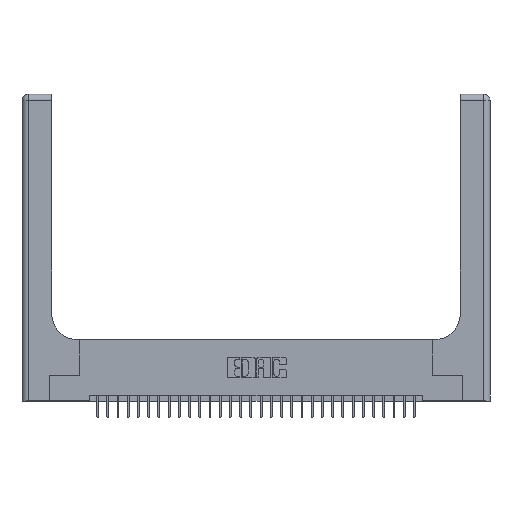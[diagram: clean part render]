
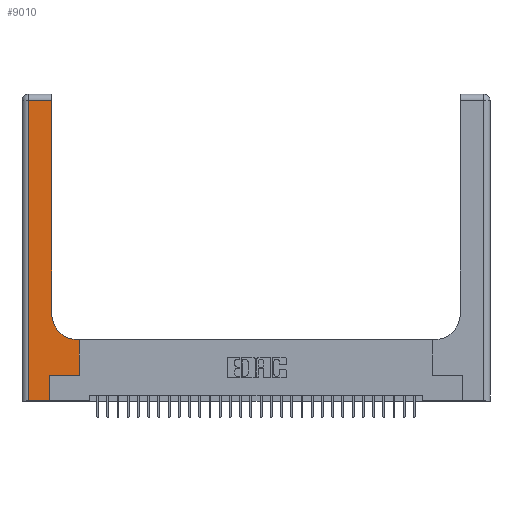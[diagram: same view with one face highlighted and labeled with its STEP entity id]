
A CAD part, top view. The second image highlights one B-rep face of the part: STEP entity #9010.
In plain terms, the highlighted planar face has unit normal (0, 0, 1).
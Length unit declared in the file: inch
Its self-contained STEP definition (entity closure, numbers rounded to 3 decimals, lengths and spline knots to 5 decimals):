
#358 = EDGE_CURVE ( 'NONE', #5891, #13282, #8172, .T. ) ;
#668 = DIRECTION ( 'NONE',  ( 0., 0., -1. ) ) ;
#2065 = DIRECTION ( 'NONE',  ( 1., 0., 0. ) ) ;
#2071 = ORIENTED_EDGE ( 'NONE', *, *, #5313, .T. ) ;
#2123 = AXIS2_PLACEMENT_3D ( 'NONE', #15393, #668, #19780 ) ;
#2156 = CARTESIAN_POINT ( 'NONE',  ( 0.269, 0., 0.37 ) ) ;
#2486 = EDGE_CURVE ( 'NONE', #23653, #8554, #8502, .T. ) ;
#2620 = LINE ( 'NONE', #26091, #23700 ) ;
#3602 = ORIENTED_EDGE ( 'NONE', *, *, #13614, .T. ) ;
#3738 = VECTOR ( 'NONE', #6688, 39.37008 ) ;
#3901 = EDGE_LOOP ( 'NONE', ( #3602, #21259, #10520, #13388, #2071, #23521, #14145, #7684, #25994 ) ) ;
#5313 = EDGE_CURVE ( 'NONE', #19761, #6849, #10259, .T. ) ;
#5891 = VERTEX_POINT ( 'NONE', #29740 ) ;
#6205 = VECTOR ( 'NONE', #19482, 39.37008 ) ;
#6592 = EDGE_CURVE ( 'NONE', #21903, #19761, #31597, .T. ) ;
#6688 = DIRECTION ( 'NONE',  ( 0., 1., 0. ) ) ;
#6849 = VERTEX_POINT ( 'NONE', #29167 ) ;
#7684 = ORIENTED_EDGE ( 'NONE', *, *, #17314, .T. ) ;
#8123 = VECTOR ( 'NONE', #10813, 39.37008 ) ;
#8172 = LINE ( 'NONE', #24734, #28862 ) ;
#8502 = LINE ( 'NONE', #12874, #8123 ) ;
#8554 = VERTEX_POINT ( 'NONE', #19736 ) ;
#9010 = ADVANCED_FACE ( 'NONE', ( #29563 ), #10465, .F. ) ;
#9840 = CARTESIAN_POINT ( 'NONE',  ( 0.269, 0., 0.37 ) ) ;
#10122 = EDGE_CURVE ( 'NONE', #13282, #21903, #19143, .T. ) ;
#10259 = LINE ( 'NONE', #2156, #3738 ) ;
#10278 = CARTESIAN_POINT ( 'NONE',  ( 0.2915, 3., 0.37 ) ) ;
#10465 = PLANE ( 'NONE',  #2123 ) ;
#10520 = ORIENTED_EDGE ( 'NONE', *, *, #10122, .T. ) ;
#10813 = DIRECTION ( 'NONE',  ( 0., 1., 0. ) ) ;
#11694 = DIRECTION ( 'NONE',  ( 1., 0., 0. ) ) ;
#12305 = CARTESIAN_POINT ( 'NONE',  ( 0.06, 3., 0.37 ) ) ;
#12601 = LINE ( 'NONE', #10278, #27867 ) ;
#12874 = CARTESIAN_POINT ( 'NONE',  ( 0.5585, 0.25, 0.37 ) ) ;
#13282 = VERTEX_POINT ( 'NONE', #31116 ) ;
#13388 = ORIENTED_EDGE ( 'NONE', *, *, #6592, .T. ) ;
#13614 = EDGE_CURVE ( 'NONE', #23960, #5891, #12601, .T. ) ;
#13869 = EDGE_CURVE ( 'NONE', #16204, #23960, #15624, .T. ) ;
#14003 = VECTOR ( 'NONE', #16223, 39.37008 ) ;
#14145 = ORIENTED_EDGE ( 'NONE', *, *, #2486, .T. ) ;
#14437 = CARTESIAN_POINT ( 'NONE',  ( 0.5415, 0.85, 0.37 ) ) ;
#15393 = CARTESIAN_POINT ( 'NONE',  ( 0., 3., 0.37 ) ) ;
#15423 = LINE ( 'NONE', #22068, #6205 ) ;
#15624 = CIRCLE ( 'NONE', #28892, 0.25 ) ;
#16204 = VERTEX_POINT ( 'NONE', #20598 ) ;
#16223 = DIRECTION ( 'NONE',  ( 1., 0., 0. ) ) ;
#16461 = VECTOR ( 'NONE', #17205, 39.37008 ) ;
#16772 = DIRECTION ( 'NONE',  ( 0., 0., -1. ) ) ;
#17205 = DIRECTION ( 'NONE',  ( 0., -1., 0. ) ) ;
#17314 = EDGE_CURVE ( 'NONE', #8554, #16204, #15423, .T. ) ;
#18265 = CARTESIAN_POINT ( 'NONE',  ( 0.2915, 0.85, 0.37 ) ) ;
#18275 = DIRECTION ( 'NONE',  ( 0., 1., 0. ) ) ;
#19143 = LINE ( 'NONE', #12305, #16461 ) ;
#19157 = EDGE_CURVE ( 'NONE', #6849, #23653, #2620, .T. ) ;
#19482 = DIRECTION ( 'NONE',  ( -1., 0., 0. ) ) ;
#19736 = CARTESIAN_POINT ( 'NONE',  ( 0.5585, 0.6, 0.37 ) ) ;
#19761 = VERTEX_POINT ( 'NONE', #9840 ) ;
#19780 = DIRECTION ( 'NONE',  ( -1., 0., 0. ) ) ;
#20598 = CARTESIAN_POINT ( 'NONE',  ( 0.5415, 0.6, 0.37 ) ) ;
#20725 = CARTESIAN_POINT ( 'NONE',  ( 0., 0., 0.37 ) ) ;
#21259 = ORIENTED_EDGE ( 'NONE', *, *, #358, .T. ) ;
#21903 = VERTEX_POINT ( 'NONE', #26254 ) ;
#22068 = CARTESIAN_POINT ( 'NONE',  ( 0.2915, 0.6, 0.37 ) ) ;
#23521 = ORIENTED_EDGE ( 'NONE', *, *, #19157, .T. ) ;
#23653 = VERTEX_POINT ( 'NONE', #29015 ) ;
#23700 = VECTOR ( 'NONE', #11694, 39.37008 ) ;
#23960 = VERTEX_POINT ( 'NONE', #18265 ) ;
#24734 = CARTESIAN_POINT ( 'NONE',  ( 0., 2.94, 0.37 ) ) ;
#25994 = ORIENTED_EDGE ( 'NONE', *, *, #13869, .T. ) ;
#26091 = CARTESIAN_POINT ( 'NONE',  ( 0.269, 0.25, 0.37 ) ) ;
#26254 = CARTESIAN_POINT ( 'NONE',  ( 0.06, 0., 0.37 ) ) ;
#27867 = VECTOR ( 'NONE', #18275, 39.37008 ) ;
#28862 = VECTOR ( 'NONE', #29356, 39.37008 ) ;
#28892 = AXIS2_PLACEMENT_3D ( 'NONE', #14437, #16772, #2065 ) ;
#29015 = CARTESIAN_POINT ( 'NONE',  ( 0.5585, 0.25, 0.37 ) ) ;
#29167 = CARTESIAN_POINT ( 'NONE',  ( 0.269, 0.25, 0.37 ) ) ;
#29356 = DIRECTION ( 'NONE',  ( -1., 0., 0. ) ) ;
#29563 = FACE_OUTER_BOUND ( 'NONE', #3901, .T. ) ;
#29740 = CARTESIAN_POINT ( 'NONE',  ( 0.2915, 2.94, 0.37 ) ) ;
#31116 = CARTESIAN_POINT ( 'NONE',  ( 0.06, 2.94, 0.37 ) ) ;
#31597 = LINE ( 'NONE', #20725, #14003 ) ;
